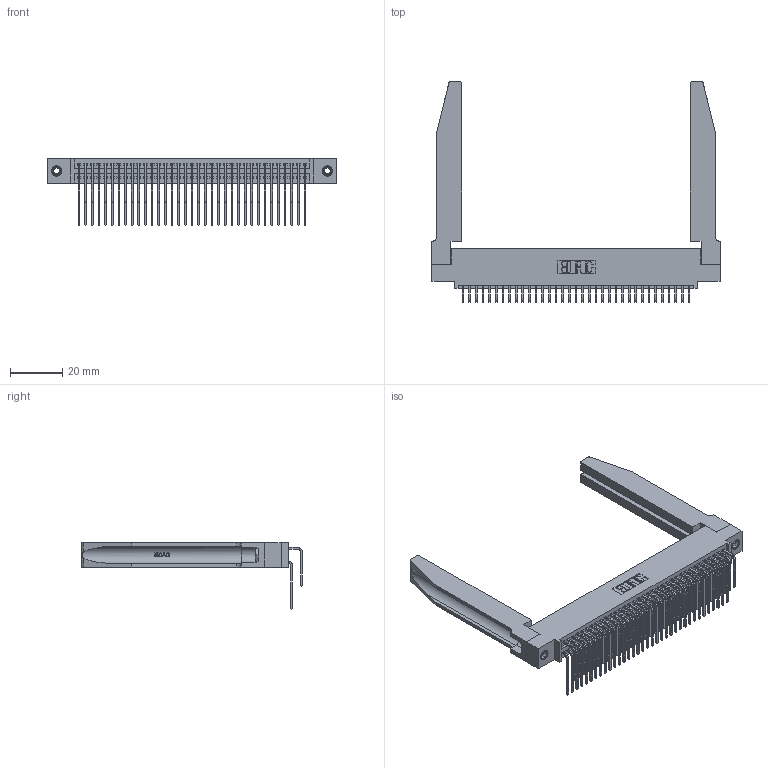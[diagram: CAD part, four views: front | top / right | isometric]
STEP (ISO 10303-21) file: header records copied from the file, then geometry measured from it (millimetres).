
FILE_DESCRIPTION (( 'STEP AP203' ), '1' );
FILE_NAME ('345-070-559-578.STEP', '2019-10-31T01:55:45', ( '' ), ( '' ), 'SwSTEP 2.0', 'SolidWorks 2016', '' );
FILE_SCHEMA (( 'CONFIG_CONTROL_DESIGN' ));
Length unit declared in the file: inch
Products named in the file (6): 345-292-001_559 Tail - 2; 345-250-001_345-250-001-102; 345-070-559-578; 345 Part_0.110 Offset - 0.156 Dia-TH; 345-292-001_558 559 Tail - 1; 345-220-078_345-220-078
Assembly tree (75 placements, depth 2):
  345-070-559-578
    345 Part_0.110 Offset - 0.156 Dia-TH
    345-292-001_558 559 Tail - 1  x35
    345-292-001_559 Tail - 2  x35
    345-250-001_345-250-001-102  x2
    345-220-078_345-220-078  x2
Bounding box: 110.13 x 84.32 x 25.53 mm (x, y, z)
Volume: 18734.5 mm3; surface area: 24901.3 mm2
Topology: 75 solids, 75 shells, 4004 faces, 11811 edges, 7770 vertices
Faces by surface type: plane 2676, cylinder 1276, bspline 36, cone 12, torus 4
Entity records: 34928 total; most frequent: CARTESIAN_POINT 6826, ORIENTED_EDGE 5606, DIRECTION 4993, EDGE_CURVE 2803, LINE 2397, VECTOR 2397, VERTEX_POINT 1860, AXIS2_PLACEMENT_3D 1298
